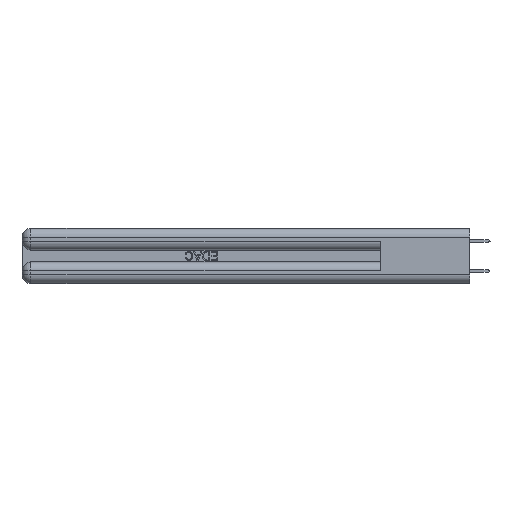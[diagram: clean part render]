
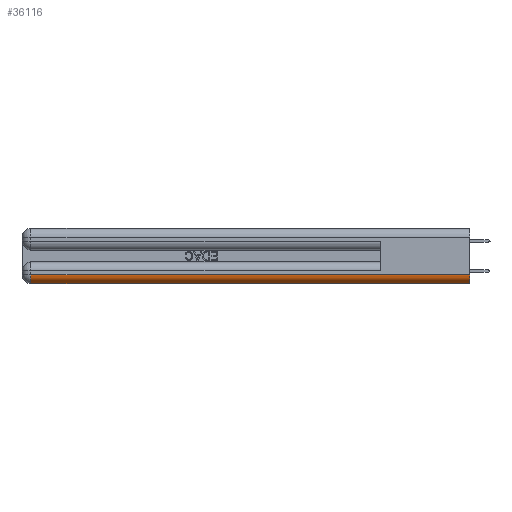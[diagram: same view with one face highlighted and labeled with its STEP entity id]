
A CAD part, left-side view. The second image highlights one B-rep face of the part: STEP entity #36116.
In plain terms, the highlighted cylindrical face has radius 1.524 mm (diameter 3.048 mm), a partial arc.
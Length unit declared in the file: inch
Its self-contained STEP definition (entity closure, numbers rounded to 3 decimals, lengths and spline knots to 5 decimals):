
#276 = VECTOR ( 'NONE', #27829, 39.37008 ) ;
#3282 = DIRECTION ( 'NONE',  ( 0., 1., 0. ) ) ;
#6134 = DIRECTION ( 'NONE',  ( 0., 0., 1. ) ) ;
#6453 = DIRECTION ( 'NONE',  ( 0., 1., 0. ) ) ;
#7618 = EDGE_CURVE ( 'NONE', #9991, #34959, #24924, .T. ) ;
#8566 = EDGE_CURVE ( 'NONE', #34662, #9991, #38614, .T. ) ;
#9846 = ORIENTED_EDGE ( 'NONE', *, *, #7618, .F. ) ;
#9991 = VERTEX_POINT ( 'NONE', #20459 ) ;
#10168 = FACE_OUTER_BOUND ( 'NONE', #18596, .T. ) ;
#10506 = EDGE_CURVE ( 'NONE', #17579, #34662, #18962, .T. ) ;
#11819 = DIRECTION ( 'NONE',  ( 0., 0., 1. ) ) ;
#17579 = VERTEX_POINT ( 'NONE', #25483 ) ;
#18014 = DIRECTION ( 'NONE',  ( 0., 1., 0. ) ) ;
#18596 = EDGE_LOOP ( 'NONE', ( #35943, #9846, #18868, #31571 ) ) ;
#18868 = ORIENTED_EDGE ( 'NONE', *, *, #8566, .F. ) ;
#18962 = LINE ( 'NONE', #28886, #39396 ) ;
#19773 = AXIS2_PLACEMENT_3D ( 'NONE', #28959, #6453, #32273 ) ;
#20459 = CARTESIAN_POINT ( 'NONE',  ( 0., 2.94, 0.06 ) ) ;
#21608 = CARTESIAN_POINT ( 'NONE',  ( 0.06, 0., 0.06 ) ) ;
#22026 = CIRCLE ( 'NONE', #25998, 0.06 ) ;
#24924 = LINE ( 'NONE', #37523, #276 ) ;
#25483 = CARTESIAN_POINT ( 'NONE',  ( 0.06, 0., 0. ) ) ;
#25998 = AXIS2_PLACEMENT_3D ( 'NONE', #21608, #40436, #6134 ) ;
#27451 = EDGE_CURVE ( 'NONE', #34959, #17579, #22026, .T. ) ;
#27731 = CARTESIAN_POINT ( 'NONE',  ( 0.06, 2.94, 0.06 ) ) ;
#27829 = DIRECTION ( 'NONE',  ( 0., -1., 0. ) ) ;
#28886 = CARTESIAN_POINT ( 'NONE',  ( 0.06, 3., 0. ) ) ;
#28959 = CARTESIAN_POINT ( 'NONE',  ( 0.06, 0., 0.06 ) ) ;
#29355 = CYLINDRICAL_SURFACE ( 'NONE', #19773, 0.06 ) ;
#30677 = AXIS2_PLACEMENT_3D ( 'NONE', #27731, #18014, #11819 ) ;
#31571 = ORIENTED_EDGE ( 'NONE', *, *, #10506, .F. ) ;
#32273 = DIRECTION ( 'NONE',  ( 0., 0., 1. ) ) ;
#32662 = CARTESIAN_POINT ( 'NONE',  ( 0.06, 2.94, 0. ) ) ;
#34662 = VERTEX_POINT ( 'NONE', #32662 ) ;
#34959 = VERTEX_POINT ( 'NONE', #39358 ) ;
#35943 = ORIENTED_EDGE ( 'NONE', *, *, #27451, .F. ) ;
#36116 = ADVANCED_FACE ( 'NONE', ( #10168 ), #29355, .T. ) ;
#37523 = CARTESIAN_POINT ( 'NONE',  ( 0., 0., 0.06 ) ) ;
#38614 = CIRCLE ( 'NONE', #30677, 0.06 ) ;
#39358 = CARTESIAN_POINT ( 'NONE',  ( 0., 0., 0.06 ) ) ;
#39396 = VECTOR ( 'NONE', #3282, 39.37008 ) ;
#40436 = DIRECTION ( 'NONE',  ( 0., -1., 0. ) ) ;
